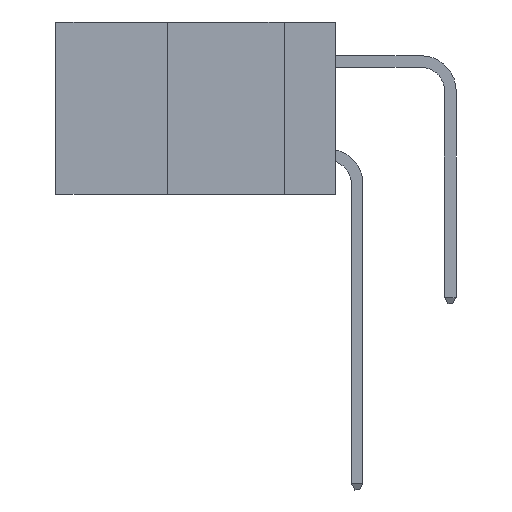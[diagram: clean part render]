
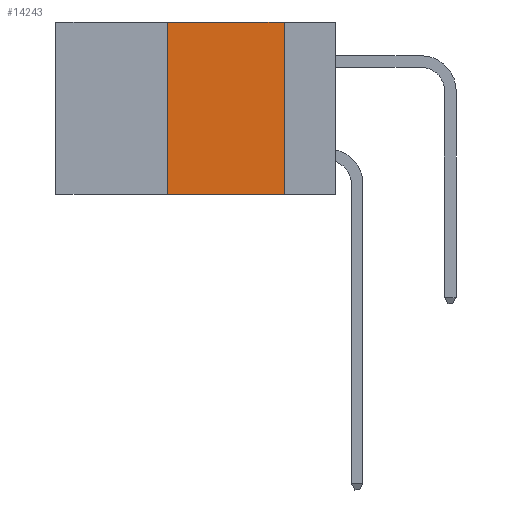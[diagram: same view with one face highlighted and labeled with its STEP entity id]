
A CAD part, left-side view. The second image highlights one B-rep face of the part: STEP entity #14243.
In plain terms, the highlighted planar face has unit normal (-1, 0, 0).
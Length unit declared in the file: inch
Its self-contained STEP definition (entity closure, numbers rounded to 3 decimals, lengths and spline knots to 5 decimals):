
#329 = EDGE_CURVE ( 'NONE', #3611, #12216, #23900, .T. ) ;
#1231 = VECTOR ( 'NONE', #11494, 39.37008 ) ;
#2089 = LINE ( 'NONE', #5674, #21193 ) ;
#2207 = ORIENTED_EDGE ( 'NONE', *, *, #17301, .F. ) ;
#3193 = DIRECTION ( 'NONE',  ( 0., 0., 1. ) ) ;
#3611 = VERTEX_POINT ( 'NONE', #5722 ) ;
#4320 = DIRECTION ( 'NONE',  ( 0., 0., -1. ) ) ;
#4861 = CARTESIAN_POINT ( 'NONE',  ( 0., 0.11, 0. ) ) ;
#5674 = CARTESIAN_POINT ( 'NONE',  ( 0., 0.11, 0. ) ) ;
#5722 = CARTESIAN_POINT ( 'NONE',  ( 0., 0.36, -0.37 ) ) ;
#5827 = ORIENTED_EDGE ( 'NONE', *, *, #329, .T. ) ;
#7941 = DIRECTION ( 'NONE',  ( 1., 0., 0. ) ) ;
#9148 = DIRECTION ( 'NONE',  ( 0., 0., -1. ) ) ;
#9246 = EDGE_CURVE ( 'NONE', #18411, #12216, #2089, .T. ) ;
#9964 = LINE ( 'NONE', #17884, #10548 ) ;
#10548 = VECTOR ( 'NONE', #3193, 39.37008 ) ;
#11252 = CARTESIAN_POINT ( 'NONE',  ( 0., 0.6, 0. ) ) ;
#11494 = DIRECTION ( 'NONE',  ( 0., -1., 0. ) ) ;
#11647 = CARTESIAN_POINT ( 'NONE',  ( 0., 0.6, 0. ) ) ;
#12216 = VERTEX_POINT ( 'NONE', #14207 ) ;
#12788 = DIRECTION ( 'NONE',  ( 0., -1., 0. ) ) ;
#13570 = LINE ( 'NONE', #11252, #1231 ) ;
#14063 = EDGE_LOOP ( 'NONE', ( #21177, #14949, #2207, #5827 ) ) ;
#14207 = CARTESIAN_POINT ( 'NONE',  ( 0., 0.11, -0.37 ) ) ;
#14235 = VECTOR ( 'NONE', #12788, 39.37008 ) ;
#14243 = ADVANCED_FACE ( 'NONE', ( #20161 ), #19288, .F. ) ;
#14247 = AXIS2_PLACEMENT_3D ( 'NONE', #11647, #7941, #4320 ) ;
#14949 = ORIENTED_EDGE ( 'NONE', *, *, #21602, .F. ) ;
#16221 = VERTEX_POINT ( 'NONE', #17185 ) ;
#17185 = CARTESIAN_POINT ( 'NONE',  ( 0., 0.36, 0. ) ) ;
#17301 = EDGE_CURVE ( 'NONE', #3611, #16221, #9964, .T. ) ;
#17884 = CARTESIAN_POINT ( 'NONE',  ( 0., 0.36, 0. ) ) ;
#18411 = VERTEX_POINT ( 'NONE', #4861 ) ;
#19288 = PLANE ( 'NONE',  #14247 ) ;
#20161 = FACE_OUTER_BOUND ( 'NONE', #14063, .T. ) ;
#21177 = ORIENTED_EDGE ( 'NONE', *, *, #9246, .F. ) ;
#21193 = VECTOR ( 'NONE', #9148, 39.37008 ) ;
#21602 = EDGE_CURVE ( 'NONE', #16221, #18411, #13570, .T. ) ;
#23900 = LINE ( 'NONE', #24043, #14235 ) ;
#24043 = CARTESIAN_POINT ( 'NONE',  ( 0., 0.6, -0.37 ) ) ;
